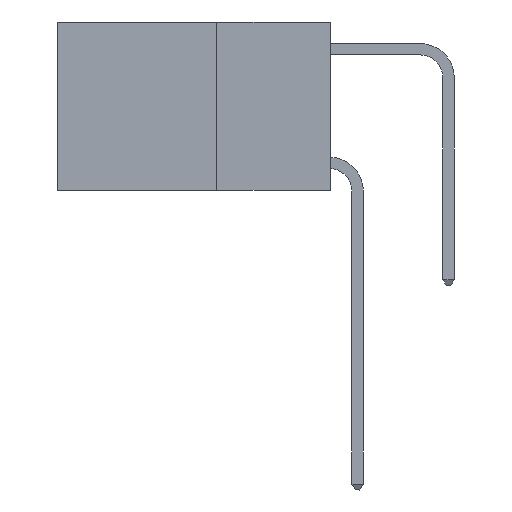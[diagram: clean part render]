
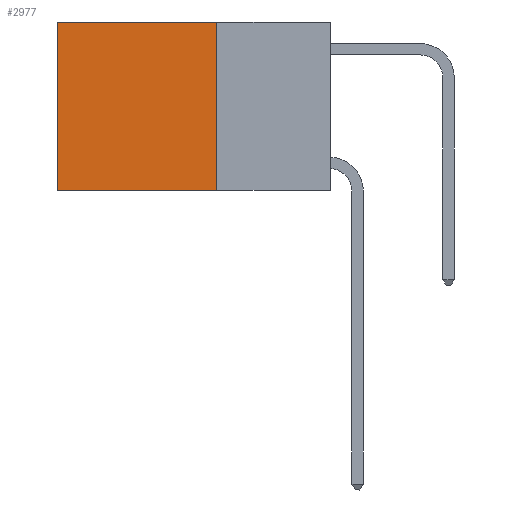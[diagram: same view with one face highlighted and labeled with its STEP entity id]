
A CAD part, left-side view. The second image highlights one B-rep face of the part: STEP entity #2977.
In plain terms, the highlighted planar face has unit normal (-1, 0, 0).
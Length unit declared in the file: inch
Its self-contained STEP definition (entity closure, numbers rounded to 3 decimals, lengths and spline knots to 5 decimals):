
#64 = VECTOR ( 'NONE', #1174, 39.37008 ) ;
#175 = LINE ( 'NONE', #5608, #64 ) ;
#501 = FACE_OUTER_BOUND ( 'NONE', #3732, .T. ) ;
#596 = EDGE_CURVE ( 'NONE', #7120, #9248, #8246, .T. ) ;
#650 = LINE ( 'NONE', #3891, #11451 ) ;
#963 = CARTESIAN_POINT ( 'NONE',  ( 0.2625, 0.6, -0.37 ) ) ;
#1006 = EDGE_CURVE ( 'NONE', #7857, #6339, #4359, .T. ) ;
#1174 = DIRECTION ( 'NONE',  ( 0., 0., -1. ) ) ;
#1418 = ORIENTED_EDGE ( 'NONE', *, *, #8876, .F. ) ;
#2126 = CARTESIAN_POINT ( 'NONE',  ( 0.2625, 0.6, 0. ) ) ;
#2977 = ADVANCED_FACE ( 'NONE', ( #501 ), #9616, .F. ) ;
#3032 = VECTOR ( 'NONE', #7553, 39.37008 ) ;
#3503 = CARTESIAN_POINT ( 'NONE',  ( 0.2625, 0.25, 0. ) ) ;
#3542 = CARTESIAN_POINT ( 'NONE',  ( 0.2625, 0.25, 0. ) ) ;
#3732 = EDGE_LOOP ( 'NONE', ( #7220, #7345, #1418, #11771 ) ) ;
#3891 = CARTESIAN_POINT ( 'NONE',  ( 0.2625, 0.6, 0. ) ) ;
#4359 = LINE ( 'NONE', #12578, #3032 ) ;
#5557 = DIRECTION ( 'NONE',  ( 0., 0., -1. ) ) ;
#5608 = CARTESIAN_POINT ( 'NONE',  ( 0.2625, 0.25, 0. ) ) ;
#6339 = VERTEX_POINT ( 'NONE', #963 ) ;
#7120 = VERTEX_POINT ( 'NONE', #3503 ) ;
#7220 = ORIENTED_EDGE ( 'NONE', *, *, #11203, .T. ) ;
#7345 = ORIENTED_EDGE ( 'NONE', *, *, #1006, .F. ) ;
#7538 = CARTESIAN_POINT ( 'NONE',  ( 0.2625, 0.25, -0.37 ) ) ;
#7553 = DIRECTION ( 'NONE',  ( 0., 1., 0. ) ) ;
#7854 = AXIS2_PLACEMENT_3D ( 'NONE', #3542, #10337, #5557 ) ;
#7857 = VERTEX_POINT ( 'NONE', #7538 ) ;
#8246 = LINE ( 'NONE', #12261, #12943 ) ;
#8876 = EDGE_CURVE ( 'NONE', #7120, #7857, #175, .T. ) ;
#9248 = VERTEX_POINT ( 'NONE', #2126 ) ;
#9305 = DIRECTION ( 'NONE',  ( 0., 1., 0. ) ) ;
#9616 = PLANE ( 'NONE',  #7854 ) ;
#10337 = DIRECTION ( 'NONE',  ( 1., 0., 0. ) ) ;
#10932 = DIRECTION ( 'NONE',  ( 0., 0., -1. ) ) ;
#11203 = EDGE_CURVE ( 'NONE', #9248, #6339, #650, .T. ) ;
#11451 = VECTOR ( 'NONE', #10932, 39.37008 ) ;
#11771 = ORIENTED_EDGE ( 'NONE', *, *, #596, .T. ) ;
#12261 = CARTESIAN_POINT ( 'NONE',  ( 0.2625, 0.25, 0. ) ) ;
#12578 = CARTESIAN_POINT ( 'NONE',  ( 0.2625, 0.25, -0.37 ) ) ;
#12943 = VECTOR ( 'NONE', #9305, 39.37008 ) ;
